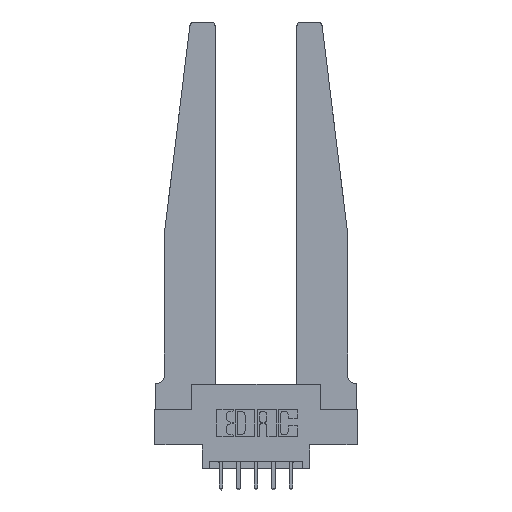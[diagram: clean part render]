
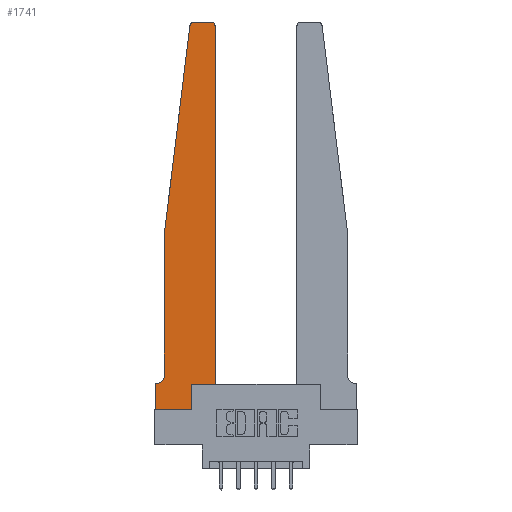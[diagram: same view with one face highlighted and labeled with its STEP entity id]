
A CAD part, top view. The second image highlights one B-rep face of the part: STEP entity #1741.
In plain terms, the highlighted planar face has unit normal (0, 0, 1).
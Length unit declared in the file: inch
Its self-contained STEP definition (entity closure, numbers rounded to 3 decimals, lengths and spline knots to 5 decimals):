
#8 = EDGE_CURVE ( 'NONE', #9153, #12175, #5514, .T. ) ;
#180 = ORIENTED_EDGE ( 'NONE', *, *, #4182, .T. ) ;
#183 = DIRECTION ( 'NONE',  ( 0., 1., 0. ) ) ;
#403 = VERTEX_POINT ( 'NONE', #3911 ) ;
#420 = VERTEX_POINT ( 'NONE', #10066 ) ;
#506 = DIRECTION ( 'NONE',  ( 1., 0., 0. ) ) ;
#655 = CARTESIAN_POINT ( 'NONE',  ( 0.395, 2.72, 0.37 ) ) ;
#704 = CIRCLE ( 'NONE', #6533, 0.03 ) ;
#873 = EDGE_LOOP ( 'NONE', ( #6974, #180, #6847, #3146, #11888, #8554, #3054, #13021, #10734, #1503, #4870, #10444 ) ) ;
#995 = EDGE_CURVE ( 'NONE', #5574, #12510, #8532, .T. ) ;
#1007 = DIRECTION ( 'NONE',  ( -1., 0., 0. ) ) ;
#1047 = VECTOR ( 'NONE', #3495, 39.37008 ) ;
#1141 = LINE ( 'NONE', #12832, #11643 ) ;
#1258 = EDGE_CURVE ( 'NONE', #12510, #420, #2916, .T. ) ;
#1343 = CARTESIAN_POINT ( 'NONE',  ( 0., 0., 0.37 ) ) ;
#1503 = ORIENTED_EDGE ( 'NONE', *, *, #995, .T. ) ;
#1631 = LINE ( 'NONE', #12181, #4659 ) ;
#1670 = DIRECTION ( 'NONE',  ( 1., 0., 0. ) ) ;
#1741 = ADVANCED_FACE ( 'NONE', ( #6262 ), #6872, .T. ) ;
#1764 = CIRCLE ( 'NONE', #7916, 0.05 ) ;
#1782 = DIRECTION ( 'NONE',  ( 0., 0., 1. ) ) ;
#1876 = EDGE_CURVE ( 'NONE', #10298, #6481, #1631, .T. ) ;
#1938 = CARTESIAN_POINT ( 'NONE',  ( 0.425, 0.18, 0.37 ) ) ;
#1956 = DIRECTION ( 'NONE',  ( -1., 0., 0. ) ) ;
#2314 = EDGE_CURVE ( 'NONE', #6402, #403, #2569, .T. ) ;
#2324 = CARTESIAN_POINT ( 'NONE',  ( 0., 0., 0.37 ) ) ;
#2360 = DIRECTION ( 'NONE',  ( 0., -1., 0. ) ) ;
#2485 = CARTESIAN_POINT ( 'NONE',  ( 0.065, 1.25, 0.37 ) ) ;
#2489 = CARTESIAN_POINT ( 'NONE',  ( 0.395, 2.75, 0.37 ) ) ;
#2569 = LINE ( 'NONE', #6015, #10705 ) ;
#2824 = CARTESIAN_POINT ( 'NONE',  ( 0.27653, 2.75, 0.37 ) ) ;
#2916 = LINE ( 'NONE', #11806, #13092 ) ;
#2963 = DIRECTION ( 'NONE',  ( 1., 0., 0. ) ) ;
#3044 = AXIS2_PLACEMENT_3D ( 'NONE', #10919, #1782, #8928 ) ;
#3054 = ORIENTED_EDGE ( 'NONE', *, *, #8, .T. ) ;
#3146 = ORIENTED_EDGE ( 'NONE', *, *, #5610, .T. ) ;
#3154 = CARTESIAN_POINT ( 'NONE',  ( 0.2605, 0., 0.37 ) ) ;
#3235 = EDGE_CURVE ( 'NONE', #10110, #5574, #5583, .T. ) ;
#3477 = CARTESIAN_POINT ( 'NONE',  ( 0.015, 0.1875, 0.37 ) ) ;
#3495 = DIRECTION ( 'NONE',  ( 0., -1., 0. ) ) ;
#3753 = CARTESIAN_POINT ( 'NONE',  ( 0., 0.1875, 0.37 ) ) ;
#3779 = AXIS2_PLACEMENT_3D ( 'NONE', #12665, #6605, #506 ) ;
#3911 = CARTESIAN_POINT ( 'NONE',  ( 0.065, 1.25, 0.37 ) ) ;
#3963 = VERTEX_POINT ( 'NONE', #10001 ) ;
#3986 = DIRECTION ( 'NONE',  ( -0.122, -0.992, 0. ) ) ;
#4106 = EDGE_CURVE ( 'NONE', #12175, #10110, #10823, .T. ) ;
#4182 = EDGE_CURVE ( 'NONE', #6481, #6402, #7015, .T. ) ;
#4659 = VECTOR ( 'NONE', #1956, 39.37008 ) ;
#4870 = ORIENTED_EDGE ( 'NONE', *, *, #1258, .T. ) ;
#5514 = LINE ( 'NONE', #1343, #10936 ) ;
#5574 = VERTEX_POINT ( 'NONE', #9587 ) ;
#5583 = LINE ( 'NONE', #7355, #10680 ) ;
#5610 = EDGE_CURVE ( 'NONE', #403, #3963, #9176, .T. ) ;
#6015 = CARTESIAN_POINT ( 'NONE',  ( 0.065, 1.25, 0.37 ) ) ;
#6262 = FACE_OUTER_BOUND ( 'NONE', #873, .T. ) ;
#6402 = VERTEX_POINT ( 'NONE', #7794 ) ;
#6481 = VERTEX_POINT ( 'NONE', #2824 ) ;
#6533 = AXIS2_PLACEMENT_3D ( 'NONE', #655, #7797, #1670 ) ;
#6605 = DIRECTION ( 'NONE',  ( 0., 0., 1. ) ) ;
#6697 = EDGE_CURVE ( 'NONE', #420, #10298, #704, .T. ) ;
#6847 = ORIENTED_EDGE ( 'NONE', *, *, #2314, .T. ) ;
#6872 = PLANE ( 'NONE',  #3044 ) ;
#6974 = ORIENTED_EDGE ( 'NONE', *, *, #1876, .T. ) ;
#7015 = CIRCLE ( 'NONE', #3779, 0.03 ) ;
#7106 = DIRECTION ( 'NONE',  ( 0., 0., -1. ) ) ;
#7355 = CARTESIAN_POINT ( 'NONE',  ( 0.2605, 0.18, 0.37 ) ) ;
#7794 = CARTESIAN_POINT ( 'NONE',  ( 0.24675, 2.72367, 0.37 ) ) ;
#7797 = DIRECTION ( 'NONE',  ( 0., 0., 1. ) ) ;
#7807 = DIRECTION ( 'NONE',  ( -1., 0., 0. ) ) ;
#7916 = AXIS2_PLACEMENT_3D ( 'NONE', #13180, #7106, #1007 ) ;
#7954 = EDGE_CURVE ( 'NONE', #12429, #9153, #1141, .T. ) ;
#8193 = CARTESIAN_POINT ( 'NONE',  ( 0., 0., 0.37 ) ) ;
#8213 = VECTOR ( 'NONE', #2963, 39.37008 ) ;
#8532 = LINE ( 'NONE', #1938, #8213 ) ;
#8554 = ORIENTED_EDGE ( 'NONE', *, *, #7954, .T. ) ;
#8729 = CARTESIAN_POINT ( 'NONE',  ( 0.425, 0.18, 0.37 ) ) ;
#8928 = DIRECTION ( 'NONE',  ( 1., 0., 0. ) ) ;
#9153 = VERTEX_POINT ( 'NONE', #3753 ) ;
#9176 = LINE ( 'NONE', #2485, #1047 ) ;
#9466 = DIRECTION ( 'NONE',  ( 1., 0., 0. ) ) ;
#9587 = CARTESIAN_POINT ( 'NONE',  ( 0.2605, 0.18, 0.37 ) ) ;
#10001 = CARTESIAN_POINT ( 'NONE',  ( 0.065, 0.2375, 0.37 ) ) ;
#10066 = CARTESIAN_POINT ( 'NONE',  ( 0.425, 2.72, 0.37 ) ) ;
#10110 = VERTEX_POINT ( 'NONE', #3154 ) ;
#10298 = VERTEX_POINT ( 'NONE', #2489 ) ;
#10444 = ORIENTED_EDGE ( 'NONE', *, *, #6697, .T. ) ;
#10680 = VECTOR ( 'NONE', #183, 39.37008 ) ;
#10705 = VECTOR ( 'NONE', #3986, 39.37008 ) ;
#10734 = ORIENTED_EDGE ( 'NONE', *, *, #3235, .T. ) ;
#10823 = LINE ( 'NONE', #2324, #13042 ) ;
#10919 = CARTESIAN_POINT ( 'NONE',  ( 0., 0.1875, 0.37 ) ) ;
#10936 = VECTOR ( 'NONE', #2360, 39.37008 ) ;
#11190 = EDGE_CURVE ( 'NONE', #3963, #12429, #1764, .T. ) ;
#11643 = VECTOR ( 'NONE', #7807, 39.37008 ) ;
#11806 = CARTESIAN_POINT ( 'NONE',  ( 0.425, 0.18, 0.37 ) ) ;
#11888 = ORIENTED_EDGE ( 'NONE', *, *, #11190, .T. ) ;
#12175 = VERTEX_POINT ( 'NONE', #8193 ) ;
#12181 = CARTESIAN_POINT ( 'NONE',  ( 0.25, 2.75, 0.37 ) ) ;
#12429 = VERTEX_POINT ( 'NONE', #3477 ) ;
#12510 = VERTEX_POINT ( 'NONE', #8729 ) ;
#12665 = CARTESIAN_POINT ( 'NONE',  ( 0.27653, 2.72, 0.37 ) ) ;
#12811 = DIRECTION ( 'NONE',  ( 0., 1., 0. ) ) ;
#12832 = CARTESIAN_POINT ( 'NONE',  ( 0.065, 0.1875, 0.37 ) ) ;
#13021 = ORIENTED_EDGE ( 'NONE', *, *, #4106, .T. ) ;
#13042 = VECTOR ( 'NONE', #9466, 39.37008 ) ;
#13092 = VECTOR ( 'NONE', #12811, 39.37008 ) ;
#13180 = CARTESIAN_POINT ( 'NONE',  ( 0.015, 0.2375, 0.37 ) ) ;
